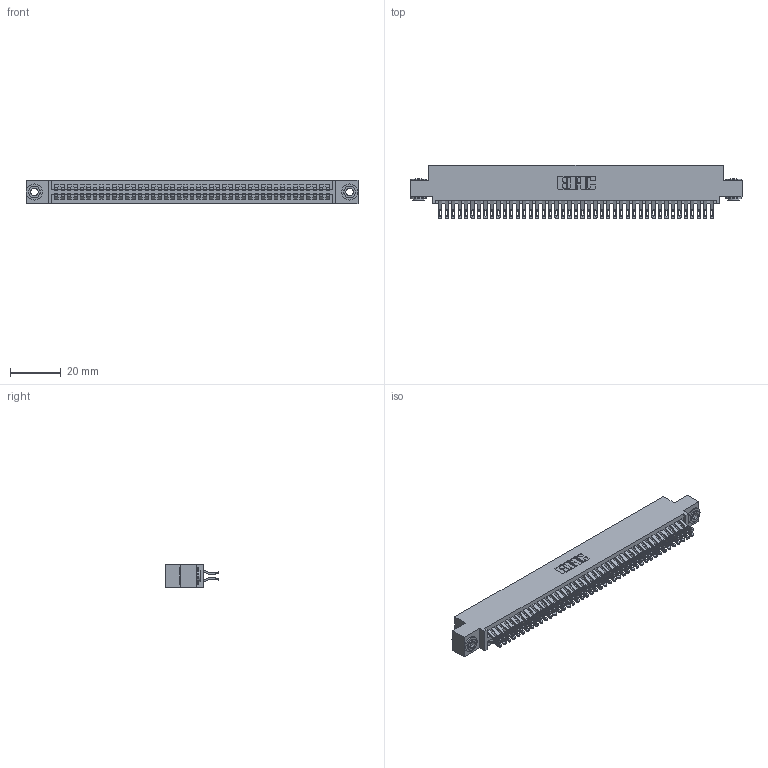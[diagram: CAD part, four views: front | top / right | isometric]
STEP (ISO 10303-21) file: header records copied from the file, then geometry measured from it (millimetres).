
FILE_DESCRIPTION (( 'STEP AP203' ), '1' );
FILE_NAME ('395-086-555-503.STEP', '2018-11-28T21:47:07', ( '' ), ( '' ), 'SwSTEP 2.0', 'SolidWorks 2016', '' );
FILE_SCHEMA (( 'CONFIG_CONTROL_DESIGN' ));
Length unit declared in the file: inch
Products named in the file (4): 345-292-001_555 Tail; 395-086-555-503; 345-250-002_345-250-002-102; 345 Part_0.110 Offset - 0.156 Dia-TH
Assembly tree (89 placements, depth 2):
  395-086-555-503
    345 Part_0.110 Offset - 0.156 Dia-TH
    345-292-001_555 Tail  x86
    345-250-002_345-250-002-102  x2
Bounding box: 130.43 x 21.13 x 9.4 mm (x, y, z)
Volume: 12874.8 mm3; surface area: 20215.8 mm2
Topology: 89 solids, 89 shells, 4984 faces, 15651 edges, 10430 vertices
Faces by surface type: plane 2760, cylinder 2216, cone 8
Entity records: 34712 total; most frequent: CARTESIAN_POINT 5829, ORIENTED_EDGE 5726, DIRECTION 5137, EDGE_CURVE 2863, LINE 2515, VECTOR 2515, VERTEX_POINT 1906, AXIS2_PLACEMENT_3D 1311
